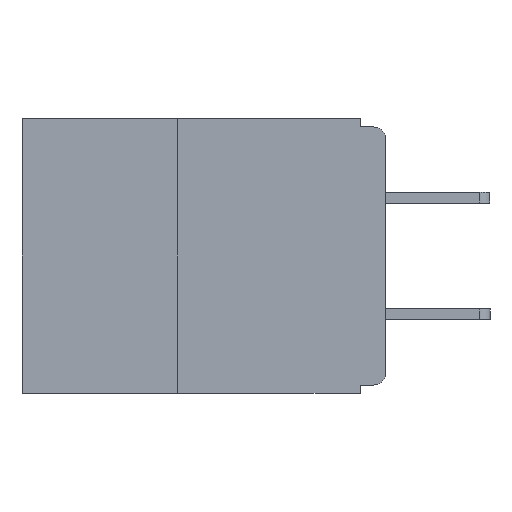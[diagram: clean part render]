
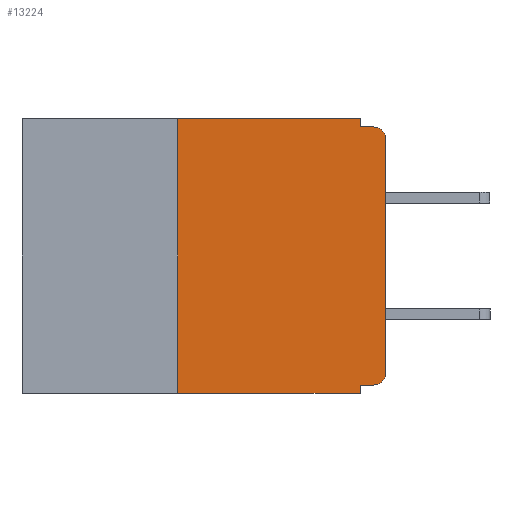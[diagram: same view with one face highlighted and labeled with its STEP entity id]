
A CAD part, left-side view. The second image highlights one B-rep face of the part: STEP entity #13224.
In plain terms, the highlighted planar face has unit normal (-1, 0, 0).
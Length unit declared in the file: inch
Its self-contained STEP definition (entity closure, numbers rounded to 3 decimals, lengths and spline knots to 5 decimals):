
#410 = VECTOR ( 'NONE', #16346, 39.37008 ) ;
#1145 = CARTESIAN_POINT ( 'NONE',  ( 0., 0.015, -0.025 ) ) ;
#1235 = CARTESIAN_POINT ( 'NONE',  ( 0., 0.015, -0.32 ) ) ;
#1331 = AXIS2_PLACEMENT_3D ( 'NONE', #14278, #3226, #16090 ) ;
#1375 = ORIENTED_EDGE ( 'NONE', *, *, #8639, .T. ) ;
#1405 = ORIENTED_EDGE ( 'NONE', *, *, #11903, .F. ) ;
#1654 = PLANE ( 'NONE',  #20212 ) ;
#1732 = DIRECTION ( 'NONE',  ( 1., 0., 0. ) ) ;
#1871 = VERTEX_POINT ( 'NONE', #3881 ) ;
#1949 = CARTESIAN_POINT ( 'NONE',  ( 0., 0., -0.01 ) ) ;
#2119 = ORIENTED_EDGE ( 'NONE', *, *, #19538, .T. ) ;
#2214 = AXIS2_PLACEMENT_3D ( 'NONE', #1145, #14175, #3109 ) ;
#2362 = VERTEX_POINT ( 'NONE', #21885 ) ;
#2861 = LINE ( 'NONE', #23228, #12141 ) ;
#2874 = LINE ( 'NONE', #13816, #12719 ) ;
#3109 = DIRECTION ( 'NONE',  ( 0., 0., -1. ) ) ;
#3226 = DIRECTION ( 'NONE',  ( -1., 0., 0. ) ) ;
#3286 = VERTEX_POINT ( 'NONE', #23235 ) ;
#3625 = VERTEX_POINT ( 'NONE', #7668 ) ;
#3881 = CARTESIAN_POINT ( 'NONE',  ( 0., 0.015, -0.01 ) ) ;
#3905 = DIRECTION ( 'NONE',  ( 0., -1., 0. ) ) ;
#4492 = LINE ( 'NONE', #20832, #8781 ) ;
#4960 = ORIENTED_EDGE ( 'NONE', *, *, #13898, .F. ) ;
#5300 = EDGE_CURVE ( 'NONE', #2362, #5704, #2861, .T. ) ;
#5704 = VERTEX_POINT ( 'NONE', #11738 ) ;
#5996 = VERTEX_POINT ( 'NONE', #1235 ) ;
#6599 = FACE_OUTER_BOUND ( 'NONE', #10807, .T. ) ;
#7375 = CARTESIAN_POINT ( 'NONE',  ( 0., 0.25, -0.33 ) ) ;
#7649 = VECTOR ( 'NONE', #23805, 39.37008 ) ;
#7668 = CARTESIAN_POINT ( 'NONE',  ( 0., 0.25, -0.33 ) ) ;
#8246 = DIRECTION ( 'NONE',  ( 0., 0., 1. ) ) ;
#8639 = EDGE_CURVE ( 'NONE', #3625, #13122, #4492, .T. ) ;
#8781 = VECTOR ( 'NONE', #11687, 39.37008 ) ;
#9074 = CARTESIAN_POINT ( 'NONE',  ( 0., 0.031, 0. ) ) ;
#9261 = VECTOR ( 'NONE', #3905, 39.37008 ) ;
#9557 = ORIENTED_EDGE ( 'NONE', *, *, #16916, .F. ) ;
#9636 = EDGE_CURVE ( 'NONE', #5996, #17384, #11925, .T. ) ;
#9798 = CIRCLE ( 'NONE', #1331, 0.015 ) ;
#10054 = CIRCLE ( 'NONE', #2214, 0.015 ) ;
#10145 = CARTESIAN_POINT ( 'NONE',  ( 0., 0.031, -0.33 ) ) ;
#10285 = VECTOR ( 'NONE', #21047, 39.37008 ) ;
#10807 = EDGE_LOOP ( 'NONE', ( #15335, #2119, #4960, #1405, #22153, #19038, #1375, #9557, #12272, #14040 ) ) ;
#10987 = DIRECTION ( 'NONE',  ( 0., 1., 0. ) ) ;
#11317 = EDGE_CURVE ( 'NONE', #15233, #3286, #2874, .T. ) ;
#11433 = LINE ( 'NONE', #10145, #10285 ) ;
#11485 = CARTESIAN_POINT ( 'NONE',  ( 0., 0.031, -0.32 ) ) ;
#11687 = DIRECTION ( 'NONE',  ( 0., -1., 0. ) ) ;
#11738 = CARTESIAN_POINT ( 'NONE',  ( 0., 0.031, 0. ) ) ;
#11903 = EDGE_CURVE ( 'NONE', #5704, #14817, #15243, .T. ) ;
#11925 = LINE ( 'NONE', #17941, #21015 ) ;
#12141 = VECTOR ( 'NONE', #23517, 39.37008 ) ;
#12272 = ORIENTED_EDGE ( 'NONE', *, *, #9636, .F. ) ;
#12404 = EDGE_CURVE ( 'NONE', #5996, #15233, #9798, .T. ) ;
#12719 = VECTOR ( 'NONE', #8246, 39.37008 ) ;
#12886 = CARTESIAN_POINT ( 'NONE',  ( 0., 0.437, 0. ) ) ;
#13122 = VERTEX_POINT ( 'NONE', #21711 ) ;
#13224 = ADVANCED_FACE ( 'NONE', ( #6599 ), #1654, .F. ) ;
#13816 = CARTESIAN_POINT ( 'NONE',  ( 0., 0., 0. ) ) ;
#13898 = EDGE_CURVE ( 'NONE', #14817, #1871, #19572, .T. ) ;
#14040 = ORIENTED_EDGE ( 'NONE', *, *, #12404, .T. ) ;
#14175 = DIRECTION ( 'NONE',  ( -1., 0., 0. ) ) ;
#14278 = CARTESIAN_POINT ( 'NONE',  ( 0., 0.015, -0.305 ) ) ;
#14696 = CARTESIAN_POINT ( 'NONE',  ( 0., 0.031, -0.01 ) ) ;
#14711 = DIRECTION ( 'NONE',  ( 0., 0., -1. ) ) ;
#14817 = VERTEX_POINT ( 'NONE', #14696 ) ;
#15233 = VERTEX_POINT ( 'NONE', #19615 ) ;
#15243 = LINE ( 'NONE', #9074, #410 ) ;
#15335 = ORIENTED_EDGE ( 'NONE', *, *, #11317, .T. ) ;
#16090 = DIRECTION ( 'NONE',  ( 0., 0., -1. ) ) ;
#16346 = DIRECTION ( 'NONE',  ( 0., 0., -1. ) ) ;
#16916 = EDGE_CURVE ( 'NONE', #17384, #13122, #11433, .T. ) ;
#17230 = EDGE_CURVE ( 'NONE', #3625, #2362, #22792, .T. ) ;
#17384 = VERTEX_POINT ( 'NONE', #11485 ) ;
#17941 = CARTESIAN_POINT ( 'NONE',  ( 0., 0., -0.32 ) ) ;
#19038 = ORIENTED_EDGE ( 'NONE', *, *, #17230, .F. ) ;
#19538 = EDGE_CURVE ( 'NONE', #3286, #1871, #10054, .T. ) ;
#19572 = LINE ( 'NONE', #1949, #9261 ) ;
#19615 = CARTESIAN_POINT ( 'NONE',  ( 0., 0., -0.305 ) ) ;
#20212 = AXIS2_PLACEMENT_3D ( 'NONE', #12886, #1732, #14711 ) ;
#20832 = CARTESIAN_POINT ( 'NONE',  ( 0., 0.437, -0.33 ) ) ;
#21015 = VECTOR ( 'NONE', #10987, 39.37008 ) ;
#21047 = DIRECTION ( 'NONE',  ( 0., 0., -1. ) ) ;
#21711 = CARTESIAN_POINT ( 'NONE',  ( 0., 0.031, -0.33 ) ) ;
#21885 = CARTESIAN_POINT ( 'NONE',  ( 0., 0.25, 0. ) ) ;
#22153 = ORIENTED_EDGE ( 'NONE', *, *, #5300, .F. ) ;
#22792 = LINE ( 'NONE', #7375, #7649 ) ;
#23228 = CARTESIAN_POINT ( 'NONE',  ( 0., 0.437, 0. ) ) ;
#23235 = CARTESIAN_POINT ( 'NONE',  ( 0., 0., -0.025 ) ) ;
#23517 = DIRECTION ( 'NONE',  ( 0., -1., 0. ) ) ;
#23805 = DIRECTION ( 'NONE',  ( 0., 0., 1. ) ) ;
